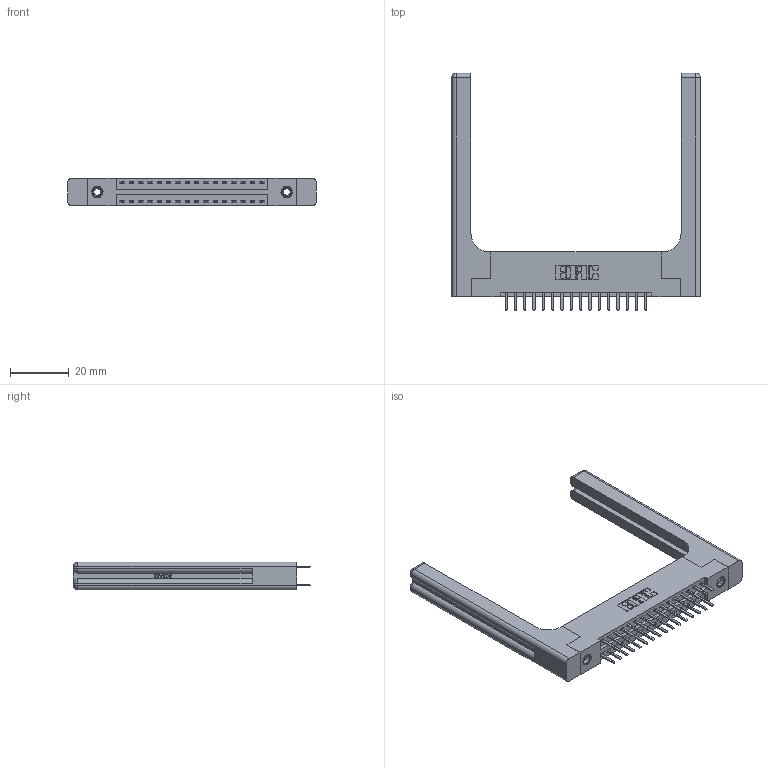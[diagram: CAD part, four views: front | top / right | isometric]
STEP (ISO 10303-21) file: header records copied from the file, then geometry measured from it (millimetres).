
FILE_DESCRIPTION (( 'STEP AP203' ), '1' );
FILE_NAME ('346-032-520-258.STEP', '2022-05-19T17:30:37', ( '' ), ( '' ), 'SwSTEP 2.0', 'SolidWorks 2020', '' );
FILE_SCHEMA (( 'CONFIG_CONTROL_DESIGN' ));
Length unit declared in the file: inch
Products named in the file (5): 346-032-520-258; 345-250-001_345-250-001-102; 346 Part_Flush Mounting Lugs - 0.156 Dia-TH; 345-292-001_345-293-120; 346-220-058_345-220-058
Assembly tree (37 placements, depth 2):
  346-032-520-258
    346 Part_Flush Mounting Lugs - 0.156 Dia-TH
    345-292-001_345-293-120  x32
    345-250-001_345-250-001-102  x2
    346-220-058_345-220-058  x2
Bounding box: 84.86 x 80.98 x 9.4 mm (x, y, z)
Volume: 15535.2 mm3; surface area: 15618.5 mm2
Topology: 37 solids, 37 shells, 2184 faces, 6247 edges, 4058 vertices
Faces by surface type: plane 1422, cylinder 702, bspline 36, cone 12, sphere 8, torus 4
Entity records: 19654 total; most frequent: CARTESIAN_POINT 4299, ORIENTED_EDGE 3016, DIRECTION 2760, EDGE_CURVE 1508, VECTOR 1216, LINE 1216, VERTEX_POINT 994, AXIS2_PLACEMENT_3D 772
